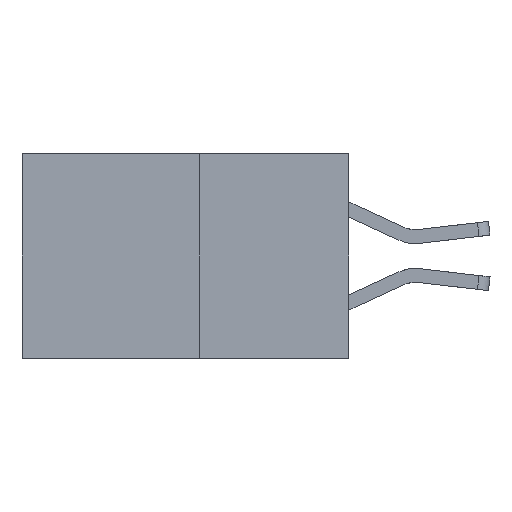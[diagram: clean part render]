
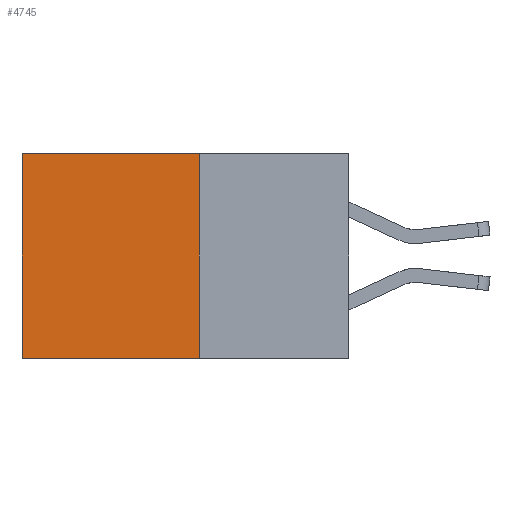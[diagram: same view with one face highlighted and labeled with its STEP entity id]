
A CAD part, left-side view. The second image highlights one B-rep face of the part: STEP entity #4745.
In plain terms, the highlighted planar face has unit normal (-1, 0, 0).
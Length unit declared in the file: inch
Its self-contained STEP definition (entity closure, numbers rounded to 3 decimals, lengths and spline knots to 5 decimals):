
#153 = VECTOR ( 'NONE', #6718, 39.37008 ) ;
#267 = LINE ( 'NONE', #2484, #5951 ) ;
#445 = DIRECTION ( 'NONE',  ( 0., 1., 0. ) ) ;
#526 = ORIENTED_EDGE ( 'NONE', *, *, #4063, .T. ) ;
#993 = CARTESIAN_POINT ( 'NONE',  ( 0.277, 0.59, -0.37 ) ) ;
#1041 = VECTOR ( 'NONE', #1811, 39.37008 ) ;
#1328 = EDGE_CURVE ( 'NONE', #5437, #7885, #5031, .T. ) ;
#1811 = DIRECTION ( 'NONE',  ( 0., 1., 0. ) ) ;
#1883 = DIRECTION ( 'NONE',  ( 0., 0., -1. ) ) ;
#2484 = CARTESIAN_POINT ( 'NONE',  ( 0.277, 0.27, -0.37 ) ) ;
#2602 = EDGE_LOOP ( 'NONE', ( #526, #8642, #2834, #7729 ) ) ;
#2631 = AXIS2_PLACEMENT_3D ( 'NONE', #7587, #7525, #7517 ) ;
#2827 = EDGE_CURVE ( 'NONE', #5437, #9055, #5643, .T. ) ;
#2834 = ORIENTED_EDGE ( 'NONE', *, *, #2827, .F. ) ;
#2880 = CARTESIAN_POINT ( 'NONE',  ( 0.277, 0.59, -0.37 ) ) ;
#3031 = EDGE_CURVE ( 'NONE', #9055, #4344, #267, .T. ) ;
#3689 = VECTOR ( 'NONE', #1883, 39.37008 ) ;
#4063 = EDGE_CURVE ( 'NONE', #7885, #4344, #7089, .T. ) ;
#4344 = VERTEX_POINT ( 'NONE', #2880 ) ;
#4745 = ADVANCED_FACE ( 'NONE', ( #7661 ), #7598, .F. ) ;
#4810 = CARTESIAN_POINT ( 'NONE',  ( 0.277, 0.27, 0. ) ) ;
#5031 = LINE ( 'NONE', #5813, #1041 ) ;
#5437 = VERTEX_POINT ( 'NONE', #4810 ) ;
#5643 = LINE ( 'NONE', #6834, #153 ) ;
#5813 = CARTESIAN_POINT ( 'NONE',  ( 0.277, 0.27, 0. ) ) ;
#5951 = VECTOR ( 'NONE', #445, 39.37008 ) ;
#6718 = DIRECTION ( 'NONE',  ( 0., 0., -1. ) ) ;
#6834 = CARTESIAN_POINT ( 'NONE',  ( 0.277, 0.27, -0.37 ) ) ;
#7089 = LINE ( 'NONE', #993, #3689 ) ;
#7517 = DIRECTION ( 'NONE',  ( 0., 0., -1. ) ) ;
#7525 = DIRECTION ( 'NONE',  ( 1., 0., 0. ) ) ;
#7587 = CARTESIAN_POINT ( 'NONE',  ( 0.277, 0.27, -0.37 ) ) ;
#7598 = PLANE ( 'NONE',  #2631 ) ;
#7661 = FACE_OUTER_BOUND ( 'NONE', #2602, .T. ) ;
#7729 = ORIENTED_EDGE ( 'NONE', *, *, #1328, .T. ) ;
#7750 = CARTESIAN_POINT ( 'NONE',  ( 0.277, 0.59, 0. ) ) ;
#7885 = VERTEX_POINT ( 'NONE', #7750 ) ;
#8642 = ORIENTED_EDGE ( 'NONE', *, *, #3031, .F. ) ;
#8832 = CARTESIAN_POINT ( 'NONE',  ( 0.277, 0.27, -0.37 ) ) ;
#9055 = VERTEX_POINT ( 'NONE', #8832 ) ;
